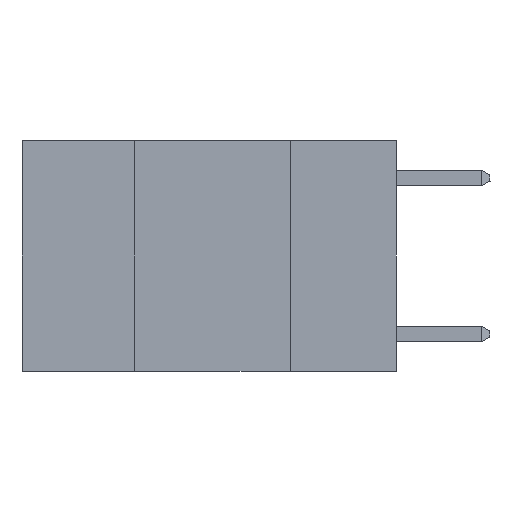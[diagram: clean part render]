
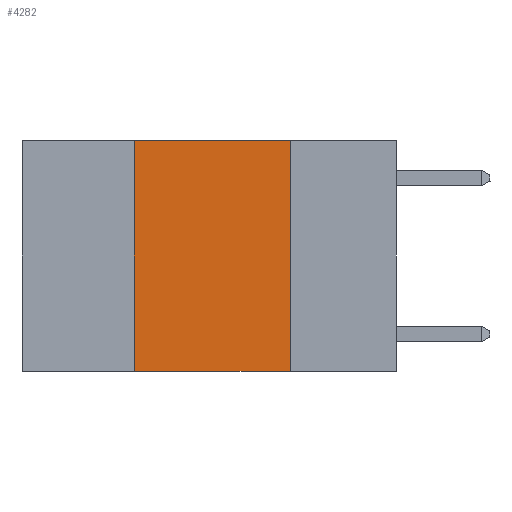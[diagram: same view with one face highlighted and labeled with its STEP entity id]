
A CAD part, left-side view. The second image highlights one B-rep face of the part: STEP entity #4282.
In plain terms, the highlighted planar face has unit normal (-1, 0, 0).
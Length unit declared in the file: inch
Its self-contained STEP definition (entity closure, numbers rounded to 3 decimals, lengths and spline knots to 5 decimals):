
#16 = ORIENTED_EDGE ( 'NONE', *, *, #9421, .F. ) ;
#110 = CARTESIAN_POINT ( 'NONE',  ( 0., 0.6, 0. ) ) ;
#114 = LINE ( 'NONE', #4755, #2237 ) ;
#487 = ORIENTED_EDGE ( 'NONE', *, *, #3110, .F. ) ;
#1142 = ORIENTED_EDGE ( 'NONE', *, *, #7564, .F. ) ;
#1323 = VERTEX_POINT ( 'NONE', #5104 ) ;
#1369 = PLANE ( 'NONE',  #5063 ) ;
#1692 = VECTOR ( 'NONE', #6553, 39.37008 ) ;
#2237 = VECTOR ( 'NONE', #4805, 39.37008 ) ;
#2258 = LINE ( 'NONE', #6590, #1692 ) ;
#2368 = CARTESIAN_POINT ( 'NONE',  ( 0., 0.17, 0. ) ) ;
#2436 = VERTEX_POINT ( 'NONE', #2845 ) ;
#2845 = CARTESIAN_POINT ( 'NONE',  ( 0., 0.42, -0.37 ) ) ;
#2914 = ORIENTED_EDGE ( 'NONE', *, *, #4944, .T. ) ;
#3110 = EDGE_CURVE ( 'NONE', #4846, #6380, #114, .T. ) ;
#3321 = FACE_OUTER_BOUND ( 'NONE', #5036, .T. ) ;
#4282 = ADVANCED_FACE ( 'NONE', ( #3321 ), #1369, .F. ) ;
#4755 = CARTESIAN_POINT ( 'NONE',  ( 0., 0.6, 0. ) ) ;
#4805 = DIRECTION ( 'NONE',  ( 0., -1., 0. ) ) ;
#4846 = VERTEX_POINT ( 'NONE', #8295 ) ;
#4925 = VECTOR ( 'NONE', #6181, 39.37008 ) ;
#4944 = EDGE_CURVE ( 'NONE', #2436, #1323, #2258, .T. ) ;
#5036 = EDGE_LOOP ( 'NONE', ( #16, #487, #1142, #2914 ) ) ;
#5063 = AXIS2_PLACEMENT_3D ( 'NONE', #110, #9970, #9940 ) ;
#5104 = CARTESIAN_POINT ( 'NONE',  ( 0., 0.17, -0.37 ) ) ;
#5293 = LINE ( 'NONE', #5800, #8239 ) ;
#5765 = DIRECTION ( 'NONE',  ( 0., 0., 1. ) ) ;
#5800 = CARTESIAN_POINT ( 'NONE',  ( 0., 0.42, 0. ) ) ;
#6181 = DIRECTION ( 'NONE',  ( 0., 0., -1. ) ) ;
#6380 = VERTEX_POINT ( 'NONE', #8480 ) ;
#6553 = DIRECTION ( 'NONE',  ( 0., -1., 0. ) ) ;
#6590 = CARTESIAN_POINT ( 'NONE',  ( 0., 0.6, -0.37 ) ) ;
#7564 = EDGE_CURVE ( 'NONE', #2436, #4846, #5293, .T. ) ;
#8239 = VECTOR ( 'NONE', #5765, 39.37008 ) ;
#8295 = CARTESIAN_POINT ( 'NONE',  ( 0., 0.42, 0. ) ) ;
#8480 = CARTESIAN_POINT ( 'NONE',  ( 0., 0.17, 0. ) ) ;
#9052 = LINE ( 'NONE', #2368, #4925 ) ;
#9421 = EDGE_CURVE ( 'NONE', #6380, #1323, #9052, .T. ) ;
#9940 = DIRECTION ( 'NONE',  ( 0., 0., -1. ) ) ;
#9970 = DIRECTION ( 'NONE',  ( 1., 0., 0. ) ) ;
